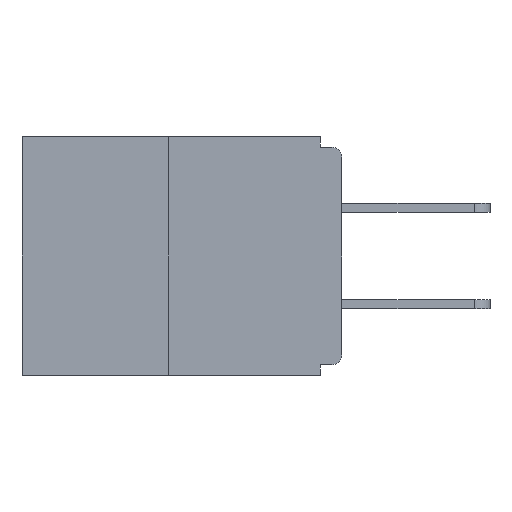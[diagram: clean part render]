
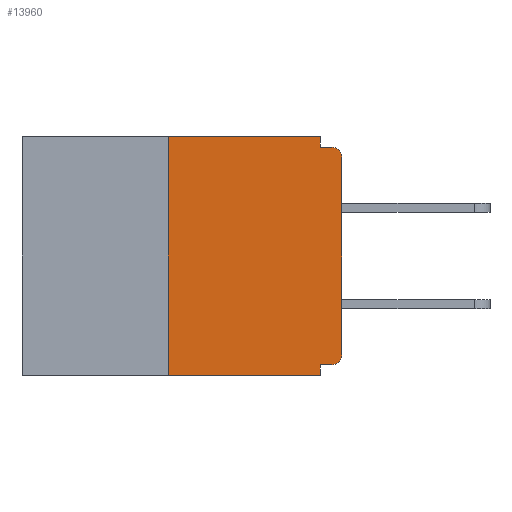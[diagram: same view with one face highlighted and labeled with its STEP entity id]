
A CAD part, left-side view. The second image highlights one B-rep face of the part: STEP entity #13960.
In plain terms, the highlighted planar face has unit normal (-1, 0, 0).
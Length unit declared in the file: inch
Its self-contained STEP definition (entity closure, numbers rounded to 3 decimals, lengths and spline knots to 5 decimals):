
#938 = LINE ( 'NONE', #10005, #9880 ) ;
#1058 = CARTESIAN_POINT ( 'NONE',  ( 0., 0.031, 0. ) ) ;
#1099 = VERTEX_POINT ( 'NONE', #17222 ) ;
#1228 = VERTEX_POINT ( 'NONE', #17636 ) ;
#1662 = DIRECTION ( 'NONE',  ( -1., 0., 0. ) ) ;
#1741 = DIRECTION ( 'NONE',  ( 0., 0., -1. ) ) ;
#1895 = VERTEX_POINT ( 'NONE', #10680 ) ;
#1973 = CARTESIAN_POINT ( 'NONE',  ( 0., 0.031, -0.343 ) ) ;
#2576 = ORIENTED_EDGE ( 'NONE', *, *, #5835, .F. ) ;
#2946 = LINE ( 'NONE', #1058, #15563 ) ;
#3479 = DIRECTION ( 'NONE',  ( 0., 0., 1. ) ) ;
#3565 = EDGE_CURVE ( 'NONE', #19846, #21329, #11219, .T. ) ;
#3602 = VERTEX_POINT ( 'NONE', #6065 ) ;
#3614 = ORIENTED_EDGE ( 'NONE', *, *, #4358, .F. ) ;
#3855 = VERTEX_POINT ( 'NONE', #14728 ) ;
#3929 = EDGE_CURVE ( 'NONE', #5469, #3602, #13845, .T. ) ;
#4059 = VECTOR ( 'NONE', #9259, 39.37008 ) ;
#4124 = EDGE_LOOP ( 'NONE', ( #4186, #14179, #9245, #18531, #12237, #12302, #12813, #15787, #3614, #2576 ) ) ;
#4186 = ORIENTED_EDGE ( 'NONE', *, *, #3565, .F. ) ;
#4358 = EDGE_CURVE ( 'NONE', #6046, #3602, #8673, .T. ) ;
#5119 = DIRECTION ( 'NONE',  ( 0., 0., -1. ) ) ;
#5127 = VECTOR ( 'NONE', #12456, 39.37008 ) ;
#5469 = VERTEX_POINT ( 'NONE', #14454 ) ;
#5631 = EDGE_CURVE ( 'NONE', #1895, #19846, #938, .T. ) ;
#5835 = EDGE_CURVE ( 'NONE', #21329, #6046, #2946, .T. ) ;
#6046 = VERTEX_POINT ( 'NONE', #16326 ) ;
#6065 = CARTESIAN_POINT ( 'NONE',  ( 0., 0.015, -0.015 ) ) ;
#7185 = EDGE_CURVE ( 'NONE', #1099, #3855, #10962, .T. ) ;
#7528 = CARTESIAN_POINT ( 'NONE',  ( 0., 0., 0. ) ) ;
#7919 = CARTESIAN_POINT ( 'NONE',  ( 0., 0.031, 0. ) ) ;
#8512 = DIRECTION ( 'NONE',  ( 0., 0., -1. ) ) ;
#8673 = LINE ( 'NONE', #20929, #4059 ) ;
#9245 = ORIENTED_EDGE ( 'NONE', *, *, #21301, .T. ) ;
#9259 = DIRECTION ( 'NONE',  ( 0., -1., 0. ) ) ;
#9880 = VECTOR ( 'NONE', #3479, 39.37008 ) ;
#9890 = CARTESIAN_POINT ( 'NONE',  ( 0., 0.015, -0.03 ) ) ;
#9901 = DIRECTION ( 'NONE',  ( 1., 0., 0. ) ) ;
#10005 = CARTESIAN_POINT ( 'NONE',  ( 0., 0.25, 0. ) ) ;
#10517 = LINE ( 'NONE', #1973, #16183 ) ;
#10680 = CARTESIAN_POINT ( 'NONE',  ( 0., 0.25, -0.343 ) ) ;
#10920 = DIRECTION ( 'NONE',  ( 0., 0., -1. ) ) ;
#10962 = LINE ( 'NONE', #16608, #17161 ) ;
#11219 = LINE ( 'NONE', #15909, #20289 ) ;
#11487 = LINE ( 'NONE', #19513, #12295 ) ;
#11523 = DIRECTION ( 'NONE',  ( -1., 0., 0. ) ) ;
#11538 = DIRECTION ( 'NONE',  ( 0., 0., -1. ) ) ;
#11646 = VERTEX_POINT ( 'NONE', #17495 ) ;
#11663 = AXIS2_PLACEMENT_3D ( 'NONE', #9890, #1662, #11538 ) ;
#11691 = DIRECTION ( 'NONE',  ( 0., 1., 0. ) ) ;
#11825 = EDGE_CURVE ( 'NONE', #1228, #5469, #15163, .T. ) ;
#12099 = CARTESIAN_POINT ( 'NONE',  ( 0., 0.25, 0. ) ) ;
#12237 = ORIENTED_EDGE ( 'NONE', *, *, #7185, .F. ) ;
#12295 = VECTOR ( 'NONE', #19371, 39.37008 ) ;
#12302 = ORIENTED_EDGE ( 'NONE', *, *, #19735, .T. ) ;
#12456 = DIRECTION ( 'NONE',  ( 0., 0., 1. ) ) ;
#12519 = AXIS2_PLACEMENT_3D ( 'NONE', #16727, #11523, #8512 ) ;
#12813 = ORIENTED_EDGE ( 'NONE', *, *, #11825, .T. ) ;
#13845 = CIRCLE ( 'NONE', #11663, 0.015 ) ;
#13960 = ADVANCED_FACE ( 'NONE', ( #19326 ), #16395, .F. ) ;
#14179 = ORIENTED_EDGE ( 'NONE', *, *, #5631, .F. ) ;
#14186 = DIRECTION ( 'NONE',  ( 0., -1., 0. ) ) ;
#14329 = EDGE_CURVE ( 'NONE', #3855, #11646, #10517, .T. ) ;
#14454 = CARTESIAN_POINT ( 'NONE',  ( 0., 0., -0.03 ) ) ;
#14728 = CARTESIAN_POINT ( 'NONE',  ( 0., 0.031, -0.328 ) ) ;
#15163 = LINE ( 'NONE', #7528, #5127 ) ;
#15563 = VECTOR ( 'NONE', #10920, 39.37008 ) ;
#15787 = ORIENTED_EDGE ( 'NONE', *, *, #3929, .T. ) ;
#15909 = CARTESIAN_POINT ( 'NONE',  ( 0., 0.46, 0. ) ) ;
#16183 = VECTOR ( 'NONE', #5119, 39.37008 ) ;
#16326 = CARTESIAN_POINT ( 'NONE',  ( 0., 0.031, -0.015 ) ) ;
#16395 = PLANE ( 'NONE',  #18809 ) ;
#16608 = CARTESIAN_POINT ( 'NONE',  ( 0., 0., -0.328 ) ) ;
#16727 = CARTESIAN_POINT ( 'NONE',  ( 0., 0.015, -0.313 ) ) ;
#17161 = VECTOR ( 'NONE', #11691, 39.37008 ) ;
#17222 = CARTESIAN_POINT ( 'NONE',  ( 0., 0.015, -0.328 ) ) ;
#17495 = CARTESIAN_POINT ( 'NONE',  ( 0., 0.031, -0.343 ) ) ;
#17636 = CARTESIAN_POINT ( 'NONE',  ( 0., 0., -0.313 ) ) ;
#18035 = CIRCLE ( 'NONE', #12519, 0.015 ) ;
#18531 = ORIENTED_EDGE ( 'NONE', *, *, #14329, .F. ) ;
#18809 = AXIS2_PLACEMENT_3D ( 'NONE', #19790, #9901, #1741 ) ;
#19326 = FACE_OUTER_BOUND ( 'NONE', #4124, .T. ) ;
#19371 = DIRECTION ( 'NONE',  ( 0., -1., 0. ) ) ;
#19513 = CARTESIAN_POINT ( 'NONE',  ( 0., 0.46, -0.343 ) ) ;
#19735 = EDGE_CURVE ( 'NONE', #1099, #1228, #18035, .T. ) ;
#19790 = CARTESIAN_POINT ( 'NONE',  ( 0., 0.46, 0. ) ) ;
#19846 = VERTEX_POINT ( 'NONE', #12099 ) ;
#20289 = VECTOR ( 'NONE', #14186, 39.37008 ) ;
#20929 = CARTESIAN_POINT ( 'NONE',  ( 0., 0., -0.015 ) ) ;
#21301 = EDGE_CURVE ( 'NONE', #1895, #11646, #11487, .T. ) ;
#21329 = VERTEX_POINT ( 'NONE', #7919 ) ;
